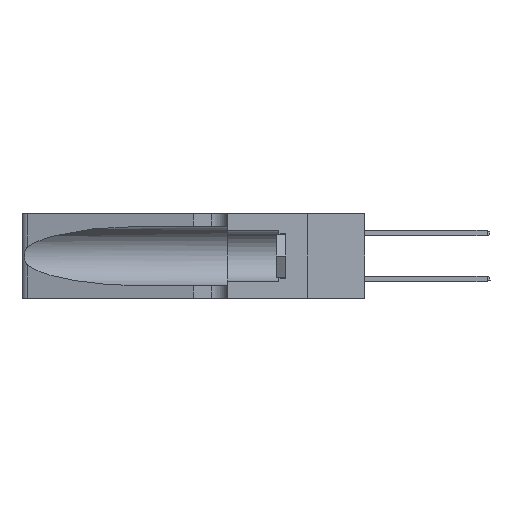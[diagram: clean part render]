
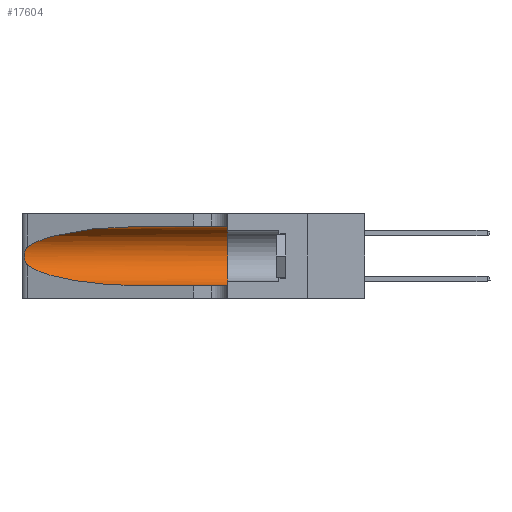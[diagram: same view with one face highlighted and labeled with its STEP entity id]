
A CAD part, left-side view. The second image highlights one B-rep face of the part: STEP entity #17604.
In plain terms, the highlighted cylindrical face has radius 3.308 mm (diameter 6.617 mm), a partial arc.
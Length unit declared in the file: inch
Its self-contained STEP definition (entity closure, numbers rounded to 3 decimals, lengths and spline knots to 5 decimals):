
#55 = CARTESIAN_POINT ( 'NONE',  ( 0.1305, 1.61858, 0.31525 ) ) ;
#894 = EDGE_CURVE ( 'NONE', #21753, #27577, #23211, .T. ) ;
#1075 = CARTESIAN_POINT ( 'NONE',  ( 0.2373, 1.15595, 0.28018 ) ) ;
#3667 = VERTEX_POINT ( 'NONE', #4718 ) ;
#4098 = CARTESIAN_POINT ( 'NONE',  ( 0.26017, 1.23833, 0.17102 ) ) ;
#4718 = CARTESIAN_POINT ( 'NONE',  ( 0.25487, 1.22718, 0.14631 ) ) ;
#5187 = CARTESIAN_POINT ( 'NONE',  ( 0.1305, 0.72297, 0.05475 ) ) ;
#5426 = VECTOR ( 'NONE', #32135, 39.37008 ) ;
#6581 = CARTESIAN_POINT ( 'NONE',  ( 0.25854, 1.2359, 0.20912 ) ) ;
#6702 = DIRECTION ( 'NONE',  ( 0., 0., -1. ) ) ;
#6965 = CARTESIAN_POINT ( 'NONE',  ( 0.1305, 1.61858, 0.185 ) ) ;
#6992 = CARTESIAN_POINT ( 'NONE',  ( 0.1305, 0.72297, 0.31525 ) ) ;
#7747 = EDGE_CURVE ( 'NONE', #22478, #3667, #9826, .T. ) ;
#9054 = CARTESIAN_POINT ( 'NONE',  ( 0.1305, 0.35, 0.31525 ) ) ;
#9222 = CARTESIAN_POINT ( 'NONE',  ( 0.26075, 1.23896, 0.19203 ) ) ;
#9570 = CARTESIAN_POINT ( 'NONE',  ( 0.1305, 0.72297, 0.05475 ) ) ;
#9826 = B_SPLINE_CURVE_WITH_KNOTS ( 'NONE', 3,
 ( #22598, #27847, #24717, #16938, #6581, #24837, #9222, #11815, #4098, #24961, #27965, #18036, #12428, #23196 ),
 .UNSPECIFIED., .F., .F.,
 ( 4, 2, 2, 2, 2, 2, 4 ),
 ( 0., 0.00027, 0.00053, 0.00107, 0.0016, 0.00187, 0.00214 ),
 .UNSPECIFIED. ) ;
#10981 =( BOUNDED_CURVE ( )  B_SPLINE_CURVE ( 3, ( #19088, #22093, #27331, #9570 ),
 .UNSPECIFIED., .F., .F. ) 
 B_SPLINE_CURVE_WITH_KNOTS ( ( 4, 4 ),
 ( 3.44316, 4.71239 ),
 .UNSPECIFIED. ) 
 CURVE ( )  GEOMETRIC_REPRESENTATION_ITEM ( )  RATIONAL_B_SPLINE_CURVE ( ( 1., 0.87, 0.87, 1. ) ) 
 REPRESENTATION_ITEM ( '' )  );
#11281 = EDGE_CURVE ( 'NONE', #19079, #16896, #26620, .T. ) ;
#11815 = CARTESIAN_POINT ( 'NONE',  ( 0.26075, 1.23896, 0.178 ) ) ;
#11882 = CARTESIAN_POINT ( 'NONE',  ( 0.1305, 0.72297, 0.31525 ) ) ;
#12417 = DIRECTION ( 'NONE',  ( 0., 1., 0. ) ) ;
#12428 = CARTESIAN_POINT ( 'NONE',  ( 0.25555, 1.22993, 0.14849 ) ) ;
#12534 = DIRECTION ( 'NONE',  ( 0., 0., 1. ) ) ;
#12650 = ORIENTED_EDGE ( 'NONE', *, *, #21915, .F. ) ;
#14007 = CARTESIAN_POINT ( 'NONE',  ( 0.1305, 0.35, 0.05475 ) ) ;
#14370 = CYLINDRICAL_SURFACE ( 'NONE', #14799, 0.13025 ) ;
#14799 = AXIS2_PLACEMENT_3D ( 'NONE', #6965, #17559, #6702 ) ;
#16123 = EDGE_LOOP ( 'NONE', ( #26170, #32782, #31040, #17520, #12650, #28428 ) ) ;
#16896 = VERTEX_POINT ( 'NONE', #14007 ) ;
#16938 = CARTESIAN_POINT ( 'NONE',  ( 0.25787, 1.23484, 0.2124 ) ) ;
#17520 = ORIENTED_EDGE ( 'NONE', *, *, #11281, .T. ) ;
#17559 = DIRECTION ( 'NONE',  ( 0., -1., 0. ) ) ;
#17604 = ADVANCED_FACE ( 'NONE', ( #31577 ), #14370, .F. ) ;
#18036 = CARTESIAN_POINT ( 'NONE',  ( 0.25639, 1.23186, 0.15144 ) ) ;
#19079 = VERTEX_POINT ( 'NONE', #5187 ) ;
#19088 = CARTESIAN_POINT ( 'NONE',  ( 0.25487, 1.22718, 0.14631 ) ) ;
#19651 = CARTESIAN_POINT ( 'NONE',  ( 0.25487, 1.22718, 0.22369 ) ) ;
#21416 = CARTESIAN_POINT ( 'NONE',  ( 0.25487, 1.22718, 0.22369 ) ) ;
#21753 = VERTEX_POINT ( 'NONE', #6992 ) ;
#21915 = EDGE_CURVE ( 'NONE', #27577, #16896, #32258, .T. ) ;
#22028 = EDGE_CURVE ( 'NONE', #21753, #22478, #23038, .T. ) ;
#22093 = CARTESIAN_POINT ( 'NONE',  ( 0.2373, 1.15595, 0.08982 ) ) ;
#22478 = VERTEX_POINT ( 'NONE', #21416 ) ;
#22598 = CARTESIAN_POINT ( 'NONE',  ( 0.25487, 1.22718, 0.22369 ) ) ;
#23038 =( BOUNDED_CURVE ( )  B_SPLINE_CURVE ( 3, ( #11882, #27541, #1075, #19651 ),
 .UNSPECIFIED., .F., .F. ) 
 B_SPLINE_CURVE_WITH_KNOTS ( ( 4, 4 ),
 ( 1.5708, 2.84003 ),
 .UNSPECIFIED. ) 
 CURVE ( )  GEOMETRIC_REPRESENTATION_ITEM ( )  RATIONAL_B_SPLINE_CURVE ( ( 1., 0.87, 0.87, 1. ) ) 
 REPRESENTATION_ITEM ( '' )  );
#23196 = CARTESIAN_POINT ( 'NONE',  ( 0.25487, 1.22718, 0.14631 ) ) ;
#23211 = LINE ( 'NONE', #55, #29235 ) ;
#24274 = AXIS2_PLACEMENT_3D ( 'NONE', #28195, #12417, #12534 ) ;
#24717 = CARTESIAN_POINT ( 'NONE',  ( 0.25639, 1.23184, 0.21858 ) ) ;
#24837 = CARTESIAN_POINT ( 'NONE',  ( 0.26018, 1.23835, 0.19895 ) ) ;
#24961 = CARTESIAN_POINT ( 'NONE',  ( 0.25856, 1.23593, 0.16098 ) ) ;
#26170 = ORIENTED_EDGE ( 'NONE', *, *, #22028, .T. ) ;
#26620 = LINE ( 'NONE', #28362, #5426 ) ;
#26745 = EDGE_CURVE ( 'NONE', #3667, #19079, #10981, .T. ) ;
#27331 = CARTESIAN_POINT ( 'NONE',  ( 0.18966, 0.96281, 0.05475 ) ) ;
#27541 = CARTESIAN_POINT ( 'NONE',  ( 0.18966, 0.96281, 0.31525 ) ) ;
#27577 = VERTEX_POINT ( 'NONE', #9054 ) ;
#27847 = CARTESIAN_POINT ( 'NONE',  ( 0.25555, 1.22994, 0.2215 ) ) ;
#27965 = CARTESIAN_POINT ( 'NONE',  ( 0.25789, 1.23486, 0.15765 ) ) ;
#28195 = CARTESIAN_POINT ( 'NONE',  ( 0.1305, 0.35, 0.185 ) ) ;
#28362 = CARTESIAN_POINT ( 'NONE',  ( 0.1305, 1.61858, 0.05475 ) ) ;
#28428 = ORIENTED_EDGE ( 'NONE', *, *, #894, .F. ) ;
#29235 = VECTOR ( 'NONE', #33785, 39.37008 ) ;
#31040 = ORIENTED_EDGE ( 'NONE', *, *, #26745, .T. ) ;
#31577 = FACE_OUTER_BOUND ( 'NONE', #16123, .T. ) ;
#32135 = DIRECTION ( 'NONE',  ( 0., -1., 0. ) ) ;
#32258 = CIRCLE ( 'NONE', #24274, 0.13025 ) ;
#32782 = ORIENTED_EDGE ( 'NONE', *, *, #7747, .T. ) ;
#33785 = DIRECTION ( 'NONE',  ( 0., -1., 0. ) ) ;
